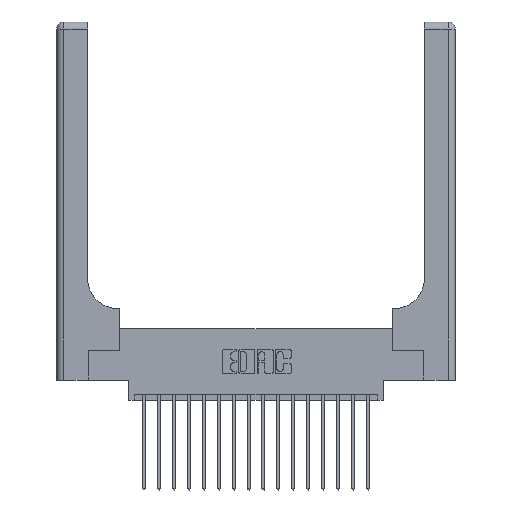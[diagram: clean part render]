
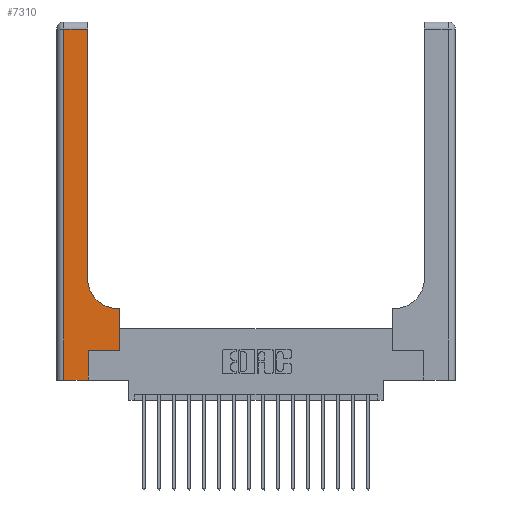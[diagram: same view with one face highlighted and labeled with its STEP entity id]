
A CAD part, top view. The second image highlights one B-rep face of the part: STEP entity #7310.
In plain terms, the highlighted planar face has unit normal (0, 0, 1).
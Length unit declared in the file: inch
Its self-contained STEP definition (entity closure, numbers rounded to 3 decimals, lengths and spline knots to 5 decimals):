
#15 = LINE ( 'NONE', #9197, #8288 ) ;
#995 = ORIENTED_EDGE ( 'NONE', *, *, #15721, .T. ) ;
#1042 = EDGE_LOOP ( 'NONE', ( #16634, #995, #15298, #12764, #4232, #1584, #15646, #14836, #11609 ) ) ;
#1530 = EDGE_CURVE ( 'NONE', #15558, #10434, #12658, .T. ) ;
#1584 = ORIENTED_EDGE ( 'NONE', *, *, #1530, .T. ) ;
#2128 = CARTESIAN_POINT ( 'NONE',  ( 0.26, 0.6, 0.37 ) ) ;
#2834 = EDGE_CURVE ( 'NONE', #6327, #16034, #11857, .T. ) ;
#2937 = CARTESIAN_POINT ( 'NONE',  ( 0.265, 0., 0.37 ) ) ;
#2971 = PLANE ( 'NONE',  #5689 ) ;
#3614 = DIRECTION ( 'NONE',  ( -1., 0., 0. ) ) ;
#3828 = VERTEX_POINT ( 'NONE', #18400 ) ;
#3913 = VECTOR ( 'NONE', #13882, 39.37008 ) ;
#4232 = ORIENTED_EDGE ( 'NONE', *, *, #12486, .T. ) ;
#4957 = CARTESIAN_POINT ( 'NONE',  ( 0.51, 0.85, 0.37 ) ) ;
#5216 = DIRECTION ( 'NONE',  ( 0., 1., 0. ) ) ;
#5689 = AXIS2_PLACEMENT_3D ( 'NONE', #9356, #13659, #7563 ) ;
#5709 = CARTESIAN_POINT ( 'NONE',  ( 0., 0., 0.37 ) ) ;
#5917 = CARTESIAN_POINT ( 'NONE',  ( 0.528, 0.25, 0.37 ) ) ;
#6150 = FACE_OUTER_BOUND ( 'NONE', #1042, .T. ) ;
#6327 = VERTEX_POINT ( 'NONE', #15527 ) ;
#6503 = CARTESIAN_POINT ( 'NONE',  ( 0.265, 0., 0.37 ) ) ;
#6588 = VERTEX_POINT ( 'NONE', #2937 ) ;
#6650 = DIRECTION ( 'NONE',  ( 0., 0., -1. ) ) ;
#7309 = AXIS2_PLACEMENT_3D ( 'NONE', #4957, #6650, #12852 ) ;
#7310 = ADVANCED_FACE ( 'NONE', ( #6150 ), #2971, .F. ) ;
#7563 = DIRECTION ( 'NONE',  ( -1., 0., 0. ) ) ;
#7577 = EDGE_CURVE ( 'NONE', #3828, #9685, #15909, .T. ) ;
#7581 = VECTOR ( 'NONE', #19185, 39.37008 ) ;
#8288 = VECTOR ( 'NONE', #16672, 39.37008 ) ;
#8558 = CARTESIAN_POINT ( 'NONE',  ( 0.06, 3., 0.37 ) ) ;
#8595 = CARTESIAN_POINT ( 'NONE',  ( 0.265, 0.25, 0.37 ) ) ;
#8894 = CARTESIAN_POINT ( 'NONE',  ( 0., 2.94, 0.37 ) ) ;
#9197 = CARTESIAN_POINT ( 'NONE',  ( 0.528, 0.25, 0.37 ) ) ;
#9298 = CARTESIAN_POINT ( 'NONE',  ( 0.26, 2.94, 0.37 ) ) ;
#9356 = CARTESIAN_POINT ( 'NONE',  ( 0., 3., 0.37 ) ) ;
#9685 = VERTEX_POINT ( 'NONE', #12512 ) ;
#9957 = VECTOR ( 'NONE', #14644, 39.37008 ) ;
#10004 = LINE ( 'NONE', #5709, #7581 ) ;
#10284 = LINE ( 'NONE', #6503, #17589 ) ;
#10393 = LINE ( 'NONE', #8894, #13542 ) ;
#10434 = VERTEX_POINT ( 'NONE', #5917 ) ;
#10606 = VECTOR ( 'NONE', #18924, 39.37008 ) ;
#10834 = EDGE_CURVE ( 'NONE', #16034, #6588, #10004, .T. ) ;
#10965 = EDGE_CURVE ( 'NONE', #10434, #19221, #15, .T. ) ;
#11261 = CARTESIAN_POINT ( 'NONE',  ( 0.265, 0.25, 0.37 ) ) ;
#11609 = ORIENTED_EDGE ( 'NONE', *, *, #7577, .T. ) ;
#11857 = LINE ( 'NONE', #8558, #9957 ) ;
#12405 = LINE ( 'NONE', #15372, #3913 ) ;
#12486 = EDGE_CURVE ( 'NONE', #6588, #15558, #10284, .T. ) ;
#12512 = CARTESIAN_POINT ( 'NONE',  ( 0.26, 0.85, 0.37 ) ) ;
#12658 = LINE ( 'NONE', #11261, #10606 ) ;
#12764 = ORIENTED_EDGE ( 'NONE', *, *, #10834, .T. ) ;
#12852 = DIRECTION ( 'NONE',  ( 1., 0., 0. ) ) ;
#13542 = VECTOR ( 'NONE', #18162, 39.37008 ) ;
#13659 = DIRECTION ( 'NONE',  ( 0., 0., -1. ) ) ;
#13866 = EDGE_CURVE ( 'NONE', #9685, #19268, #12405, .T. ) ;
#13882 = DIRECTION ( 'NONE',  ( 0., 1., 0. ) ) ;
#13979 = CARTESIAN_POINT ( 'NONE',  ( 0.528, 0.6, 0.37 ) ) ;
#14644 = DIRECTION ( 'NONE',  ( 0., -1., 0. ) ) ;
#14836 = ORIENTED_EDGE ( 'NONE', *, *, #15007, .T. ) ;
#15007 = EDGE_CURVE ( 'NONE', #19221, #3828, #17382, .T. ) ;
#15298 = ORIENTED_EDGE ( 'NONE', *, *, #2834, .T. ) ;
#15372 = CARTESIAN_POINT ( 'NONE',  ( 0.26, 3., 0.37 ) ) ;
#15527 = CARTESIAN_POINT ( 'NONE',  ( 0.06, 2.94, 0.37 ) ) ;
#15558 = VERTEX_POINT ( 'NONE', #8595 ) ;
#15646 = ORIENTED_EDGE ( 'NONE', *, *, #10965, .T. ) ;
#15721 = EDGE_CURVE ( 'NONE', #19268, #6327, #10393, .T. ) ;
#15909 = CIRCLE ( 'NONE', #7309, 0.25 ) ;
#16034 = VERTEX_POINT ( 'NONE', #16151 ) ;
#16151 = CARTESIAN_POINT ( 'NONE',  ( 0.06, 0., 0.37 ) ) ;
#16634 = ORIENTED_EDGE ( 'NONE', *, *, #13866, .T. ) ;
#16672 = DIRECTION ( 'NONE',  ( 0., 1., 0. ) ) ;
#17382 = LINE ( 'NONE', #2128, #17974 ) ;
#17589 = VECTOR ( 'NONE', #5216, 39.37008 ) ;
#17974 = VECTOR ( 'NONE', #3614, 39.37008 ) ;
#18162 = DIRECTION ( 'NONE',  ( -1., 0., 0. ) ) ;
#18400 = CARTESIAN_POINT ( 'NONE',  ( 0.51, 0.6, 0.37 ) ) ;
#18924 = DIRECTION ( 'NONE',  ( 1., 0., 0. ) ) ;
#19185 = DIRECTION ( 'NONE',  ( 1., 0., 0. ) ) ;
#19221 = VERTEX_POINT ( 'NONE', #13979 ) ;
#19268 = VERTEX_POINT ( 'NONE', #9298 ) ;
